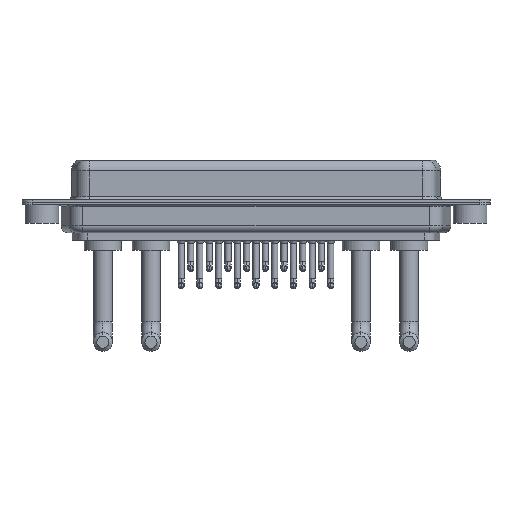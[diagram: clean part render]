
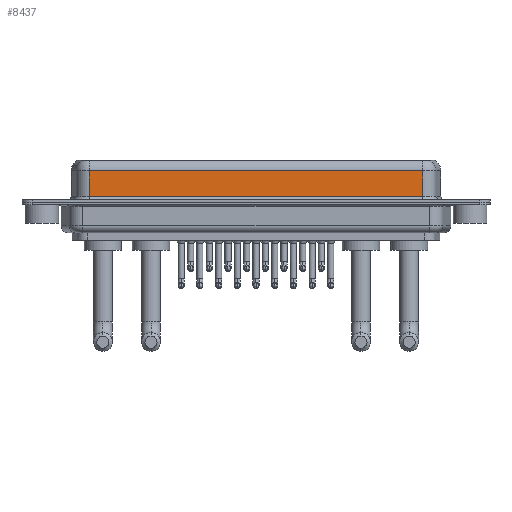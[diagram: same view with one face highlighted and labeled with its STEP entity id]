
A CAD part, front view. The second image highlights one B-rep face of the part: STEP entity #8437.
In plain terms, the highlighted planar face has unit normal (0, -1, 0).
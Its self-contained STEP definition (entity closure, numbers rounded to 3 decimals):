
#440 = VECTOR ( 'NONE', #15657, 1000. ) ;
#830 = CARTESIAN_POINT ( 'NONE',  ( 56.462, -3.95, 0.9 ) ) ;
#1374 = DIRECTION ( 'NONE',  ( 0., 0., 1. ) ) ;
#1541 = VERTEX_POINT ( 'NONE', #15139 ) ;
#1675 = DIRECTION ( 'NONE',  ( 1., 0., 0. ) ) ;
#1724 = DIRECTION ( 'NONE',  ( 0., 0., -1. ) ) ;
#2821 = VECTOR ( 'NONE', #1724, 1000. ) ;
#2897 = EDGE_CURVE ( 'NONE', #4169, #19857, #6908, .T. ) ;
#3370 = CARTESIAN_POINT ( 'NONE',  ( 7.038, -3.95, 6.4 ) ) ;
#3947 = AXIS2_PLACEMENT_3D ( 'NONE', #13302, #16551, #1374 ) ;
#4169 = VERTEX_POINT ( 'NONE', #16646 ) ;
#4788 = DIRECTION ( 'NONE',  ( -1., 0., 0. ) ) ;
#6842 = CARTESIAN_POINT ( 'NONE',  ( 56.462, -3.95, 6.4 ) ) ;
#6908 = LINE ( 'NONE', #13713, #19466 ) ;
#8437 = ADVANCED_FACE ( 'NONE', ( #12862 ), #19789, .F. ) ;
#10024 = VERTEX_POINT ( 'NONE', #830 ) ;
#10079 = ORIENTED_EDGE ( 'NONE', *, *, #11976, .T. ) ;
#10582 = EDGE_LOOP ( 'NONE', ( #17840, #20448, #12340, #10079 ) ) ;
#11179 = EDGE_CURVE ( 'NONE', #19857, #1541, #12316, .T. ) ;
#11976 = EDGE_CURVE ( 'NONE', #1541, #10024, #12150, .T. ) ;
#12150 = LINE ( 'NONE', #20404, #12825 ) ;
#12316 = LINE ( 'NONE', #3370, #2821 ) ;
#12340 = ORIENTED_EDGE ( 'NONE', *, *, #11179, .T. ) ;
#12825 = VECTOR ( 'NONE', #1675, 1000. ) ;
#12862 = FACE_OUTER_BOUND ( 'NONE', #10582, .T. ) ;
#13302 = CARTESIAN_POINT ( 'NONE',  ( 56.462, -3.95, 6.4 ) ) ;
#13713 = CARTESIAN_POINT ( 'NONE',  ( 56.462, -3.95, 4.65 ) ) ;
#15139 = CARTESIAN_POINT ( 'NONE',  ( 7.038, -3.95, 0.9 ) ) ;
#15657 = DIRECTION ( 'NONE',  ( 0., 0., -1. ) ) ;
#16088 = CARTESIAN_POINT ( 'NONE',  ( 7.038, -3.95, 4.65 ) ) ;
#16152 = EDGE_CURVE ( 'NONE', #4169, #10024, #20451, .T. ) ;
#16551 = DIRECTION ( 'NONE',  ( 0., 1., 0. ) ) ;
#16646 = CARTESIAN_POINT ( 'NONE',  ( 56.462, -3.95, 4.65 ) ) ;
#17840 = ORIENTED_EDGE ( 'NONE', *, *, #16152, .F. ) ;
#19466 = VECTOR ( 'NONE', #4788, 1000. ) ;
#19789 = PLANE ( 'NONE',  #3947 ) ;
#19857 = VERTEX_POINT ( 'NONE', #16088 ) ;
#20404 = CARTESIAN_POINT ( 'NONE',  ( 56.462, -3.95, 0.9 ) ) ;
#20448 = ORIENTED_EDGE ( 'NONE', *, *, #2897, .T. ) ;
#20451 = LINE ( 'NONE', #6842, #440 ) ;
